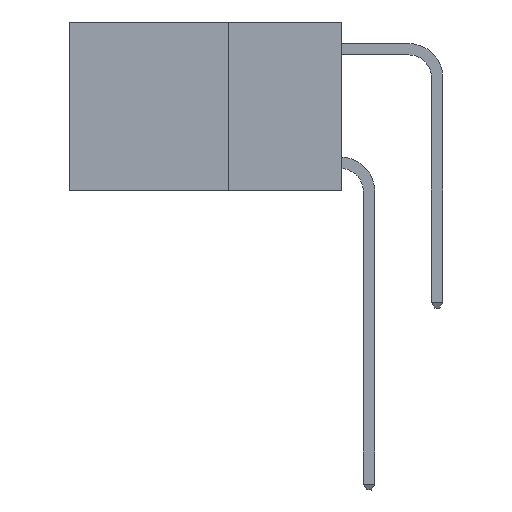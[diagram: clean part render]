
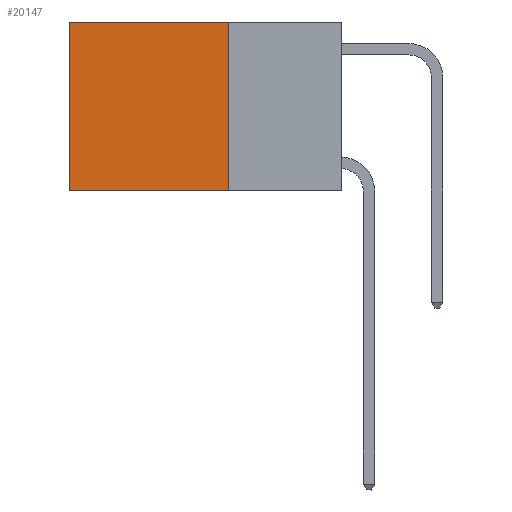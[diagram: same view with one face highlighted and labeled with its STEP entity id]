
A CAD part, left-side view. The second image highlights one B-rep face of the part: STEP entity #20147.
In plain terms, the highlighted planar face has unit normal (-1, 0, 0).
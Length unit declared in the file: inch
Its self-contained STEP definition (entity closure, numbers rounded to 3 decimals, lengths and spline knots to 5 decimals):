
#912 = LINE ( 'NONE', #1142, #4764 ) ;
#1142 = CARTESIAN_POINT ( 'NONE',  ( 0.2625, 0.6, 0. ) ) ;
#1889 = CARTESIAN_POINT ( 'NONE',  ( 0.2625, 0.25, 0. ) ) ;
#4140 = VERTEX_POINT ( 'NONE', #22135 ) ;
#4658 = EDGE_CURVE ( 'NONE', #9912, #4140, #24700, .T. ) ;
#4764 = VECTOR ( 'NONE', #8151, 39.37008 ) ;
#5813 = ORIENTED_EDGE ( 'NONE', *, *, #4658, .F. ) ;
#6825 = CARTESIAN_POINT ( 'NONE',  ( 0.2625, 0.25, 0. ) ) ;
#7432 = DIRECTION ( 'NONE',  ( 0., 0., -1. ) ) ;
#7753 = EDGE_CURVE ( 'NONE', #14112, #14040, #912, .T. ) ;
#8151 = DIRECTION ( 'NONE',  ( 0., 0., -1. ) ) ;
#9187 = ORIENTED_EDGE ( 'NONE', *, *, #15734, .T. ) ;
#9912 = VERTEX_POINT ( 'NONE', #15217 ) ;
#10111 = CARTESIAN_POINT ( 'NONE',  ( 0.2625, 0.25, 0. ) ) ;
#10680 = VECTOR ( 'NONE', #14238, 39.37008 ) ;
#12740 = FACE_OUTER_BOUND ( 'NONE', #29184, .T. ) ;
#13306 = AXIS2_PLACEMENT_3D ( 'NONE', #10111, #19658, #7432 ) ;
#14040 = VERTEX_POINT ( 'NONE', #25587 ) ;
#14112 = VERTEX_POINT ( 'NONE', #28100 ) ;
#14238 = DIRECTION ( 'NONE',  ( 0., 1., 0. ) ) ;
#14248 = DIRECTION ( 'NONE',  ( 0., 0., -1. ) ) ;
#15217 = CARTESIAN_POINT ( 'NONE',  ( 0.2625, 0.25, 0. ) ) ;
#15605 = LINE ( 'NONE', #21153, #28451 ) ;
#15734 = EDGE_CURVE ( 'NONE', #9912, #14112, #31957, .T. ) ;
#17121 = EDGE_CURVE ( 'NONE', #4140, #14040, #15605, .T. ) ;
#19658 = DIRECTION ( 'NONE',  ( 1., 0., 0. ) ) ;
#20147 = ADVANCED_FACE ( 'NONE', ( #12740 ), #27165, .F. ) ;
#21153 = CARTESIAN_POINT ( 'NONE',  ( 0.2625, 0.25, -0.37 ) ) ;
#22135 = CARTESIAN_POINT ( 'NONE',  ( 0.2625, 0.25, -0.37 ) ) ;
#23205 = ORIENTED_EDGE ( 'NONE', *, *, #17121, .F. ) ;
#23548 = VECTOR ( 'NONE', #14248, 39.37008 ) ;
#24700 = LINE ( 'NONE', #1889, #23548 ) ;
#25523 = ORIENTED_EDGE ( 'NONE', *, *, #7753, .T. ) ;
#25587 = CARTESIAN_POINT ( 'NONE',  ( 0.2625, 0.6, -0.37 ) ) ;
#27165 = PLANE ( 'NONE',  #13306 ) ;
#28100 = CARTESIAN_POINT ( 'NONE',  ( 0.2625, 0.6, 0. ) ) ;
#28270 = DIRECTION ( 'NONE',  ( 0., 1., 0. ) ) ;
#28451 = VECTOR ( 'NONE', #28270, 39.37008 ) ;
#29184 = EDGE_LOOP ( 'NONE', ( #25523, #23205, #5813, #9187 ) ) ;
#31957 = LINE ( 'NONE', #6825, #10680 ) ;
